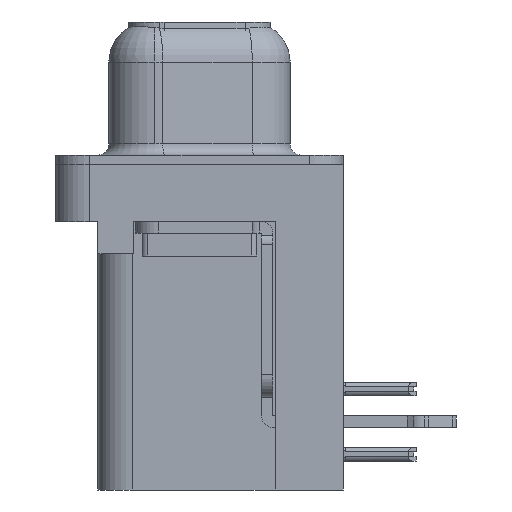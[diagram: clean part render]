
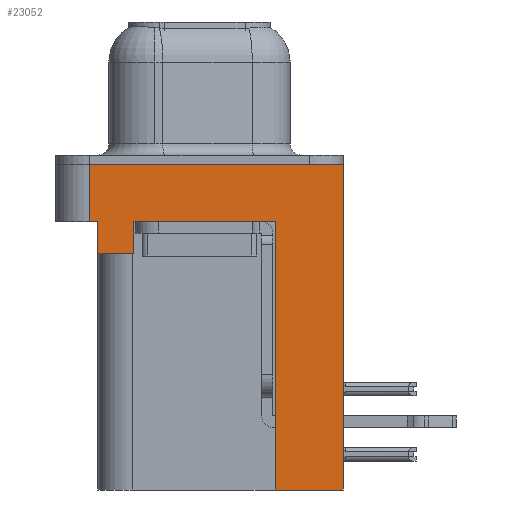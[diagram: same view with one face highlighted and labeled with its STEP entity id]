
A CAD part, left-side view. The second image highlights one B-rep face of the part: STEP entity #23052.
In plain terms, the highlighted planar face has unit normal (-1, 0, 0).
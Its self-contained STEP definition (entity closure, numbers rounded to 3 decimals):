
#307 = AXIS2_PLACEMENT_3D ( 'NONE', #25552, #6723, #23627 ) ;
#514 = LINE ( 'NONE', #6570, #21068 ) ;
#877 = ORIENTED_EDGE ( 'NONE', *, *, #11255, .T. ) ;
#1137 = ORIENTED_EDGE ( 'NONE', *, *, #2089, .F. ) ;
#1273 = CARTESIAN_POINT ( 'NONE',  ( -2.935, 4.425, -3.9 ) ) ;
#1333 = EDGE_CURVE ( 'NONE', #16677, #9877, #20522, .T. ) ;
#1867 = LINE ( 'NONE', #3802, #9758 ) ;
#2089 = EDGE_CURVE ( 'NONE', #12171, #19227, #1867, .T. ) ;
#2600 = DIRECTION ( 'NONE',  ( 0., 1., 0. ) ) ;
#3802 = CARTESIAN_POINT ( 'NONE',  ( -2.935, 4.425, -3.9 ) ) ;
#4751 = EDGE_CURVE ( 'NONE', #18012, #16927, #514, .T. ) ;
#4778 = LINE ( 'NONE', #9320, #17179 ) ;
#4952 = CARTESIAN_POINT ( 'NONE',  ( -2.935, -3.295, -2.5 ) ) ;
#5149 = CARTESIAN_POINT ( 'NONE',  ( -2.935, -6.275, -2.5 ) ) ;
#5447 = VERTEX_POINT ( 'NONE', #4952 ) ;
#5500 = VECTOR ( 'NONE', #6927, 1000. ) ;
#5755 = VECTOR ( 'NONE', #26190, 1000. ) ;
#6570 = CARTESIAN_POINT ( 'NONE',  ( -2.935, 4.775, -2.5 ) ) ;
#6723 = DIRECTION ( 'NONE',  ( -1., 0., 0. ) ) ;
#6927 = DIRECTION ( 'NONE',  ( 0., 0., 1. ) ) ;
#6999 = EDGE_CURVE ( 'NONE', #23476, #8941, #16960, .T. ) ;
#8941 = VERTEX_POINT ( 'NONE', #23737 ) ;
#9320 = CARTESIAN_POINT ( 'NONE',  ( -2.935, -3.295, -14.2 ) ) ;
#9472 = VERTEX_POINT ( 'NONE', #14575 ) ;
#9758 = VECTOR ( 'NONE', #22486, 1000. ) ;
#9877 = VERTEX_POINT ( 'NONE', #11260 ) ;
#9937 = LINE ( 'NONE', #1273, #11582 ) ;
#10074 = CARTESIAN_POINT ( 'NONE',  ( -2.935, 4.425, -2.5 ) ) ;
#10126 = ORIENTED_EDGE ( 'NONE', *, *, #20276, .F. ) ;
#10211 = ORIENTED_EDGE ( 'NONE', *, *, #13987, .T. ) ;
#10552 = ORIENTED_EDGE ( 'NONE', *, *, #11247, .F. ) ;
#10840 = FACE_OUTER_BOUND ( 'NONE', #21585, .T. ) ;
#10875 = ORIENTED_EDGE ( 'NONE', *, *, #1333, .T. ) ;
#11247 = EDGE_CURVE ( 'NONE', #9472, #5447, #14673, .T. ) ;
#11255 = EDGE_CURVE ( 'NONE', #9877, #5447, #18526, .T. ) ;
#11260 = CARTESIAN_POINT ( 'NONE',  ( -2.935, 2.895, -2.5 ) ) ;
#11582 = VECTOR ( 'NONE', #18306, 1000. ) ;
#12171 = VERTEX_POINT ( 'NONE', #18700 ) ;
#12395 = VECTOR ( 'NONE', #16980, 1000. ) ;
#13987 = EDGE_CURVE ( 'NONE', #18012, #19227, #25540, .T. ) ;
#13988 = VECTOR ( 'NONE', #22932, 1000. ) ;
#14063 = ORIENTED_EDGE ( 'NONE', *, *, #4751, .F. ) ;
#14575 = CARTESIAN_POINT ( 'NONE',  ( -2.935, -3.295, -14.2 ) ) ;
#14673 = LINE ( 'NONE', #16871, #25839 ) ;
#14892 = CARTESIAN_POINT ( 'NONE',  ( -2.935, 4.775, 0. ) ) ;
#15244 = EDGE_CURVE ( 'NONE', #23476, #9472, #4778, .T. ) ;
#16677 = VERTEX_POINT ( 'NONE', #23721 ) ;
#16871 = CARTESIAN_POINT ( 'NONE',  ( -2.935, -3.295, -14.2 ) ) ;
#16927 = VERTEX_POINT ( 'NONE', #14892 ) ;
#16960 = LINE ( 'NONE', #25760, #5500 ) ;
#16980 = DIRECTION ( 'NONE',  ( 0., -1., 0. ) ) ;
#17159 = PLANE ( 'NONE',  #307 ) ;
#17179 = VECTOR ( 'NONE', #2600, 1000. ) ;
#18012 = VERTEX_POINT ( 'NONE', #20479 ) ;
#18306 = DIRECTION ( 'NONE',  ( 0., 1., 0. ) ) ;
#18526 = LINE ( 'NONE', #22797, #13988 ) ;
#18628 = EDGE_CURVE ( 'NONE', #16927, #8941, #24979, .T. ) ;
#18700 = CARTESIAN_POINT ( 'NONE',  ( -2.935, 4.425, -3.9 ) ) ;
#19227 = VERTEX_POINT ( 'NONE', #10074 ) ;
#19598 = CARTESIAN_POINT ( 'NONE',  ( -2.935, -6.275, -14.2 ) ) ;
#20276 = EDGE_CURVE ( 'NONE', #16677, #12171, #9937, .T. ) ;
#20479 = CARTESIAN_POINT ( 'NONE',  ( -2.935, 4.775, -2.5 ) ) ;
#20522 = LINE ( 'NONE', #22725, #24644 ) ;
#21068 = VECTOR ( 'NONE', #23218, 1000. ) ;
#21095 = ORIENTED_EDGE ( 'NONE', *, *, #18628, .F. ) ;
#21585 = EDGE_LOOP ( 'NONE', ( #21095, #14063, #10211, #1137, #10126, #10875, #877, #10552, #25365, #22101 ) ) ;
#22101 = ORIENTED_EDGE ( 'NONE', *, *, #6999, .T. ) ;
#22486 = DIRECTION ( 'NONE',  ( 0., 0., 1. ) ) ;
#22725 = CARTESIAN_POINT ( 'NONE',  ( -2.935, 2.895, -3.9 ) ) ;
#22797 = CARTESIAN_POINT ( 'NONE',  ( -2.935, -6.275, -2.5 ) ) ;
#22932 = DIRECTION ( 'NONE',  ( 0., -1., 0. ) ) ;
#23052 = ADVANCED_FACE ( 'NONE', ( #10840 ), #17159, .T. ) ;
#23218 = DIRECTION ( 'NONE',  ( 0., 0., 1. ) ) ;
#23476 = VERTEX_POINT ( 'NONE', #19598 ) ;
#23627 = DIRECTION ( 'NONE',  ( 0., 0., 1. ) ) ;
#23721 = CARTESIAN_POINT ( 'NONE',  ( -2.935, 2.895, -3.9 ) ) ;
#23737 = CARTESIAN_POINT ( 'NONE',  ( -2.935, -6.275, 0. ) ) ;
#24644 = VECTOR ( 'NONE', #26582, 1000. ) ;
#24979 = LINE ( 'NONE', #27058, #12395 ) ;
#25132 = DIRECTION ( 'NONE',  ( 0., 0., 1. ) ) ;
#25365 = ORIENTED_EDGE ( 'NONE', *, *, #15244, .F. ) ;
#25540 = LINE ( 'NONE', #5149, #5755 ) ;
#25552 = CARTESIAN_POINT ( 'NONE',  ( -2.935, -6.275, -2.5 ) ) ;
#25760 = CARTESIAN_POINT ( 'NONE',  ( -2.935, -6.275, -2.5 ) ) ;
#25839 = VECTOR ( 'NONE', #25132, 1000. ) ;
#26190 = DIRECTION ( 'NONE',  ( 0., -1., 0. ) ) ;
#26582 = DIRECTION ( 'NONE',  ( 0., 0., 1. ) ) ;
#27058 = CARTESIAN_POINT ( 'NONE',  ( -2.935, -6.275, 0. ) ) ;
